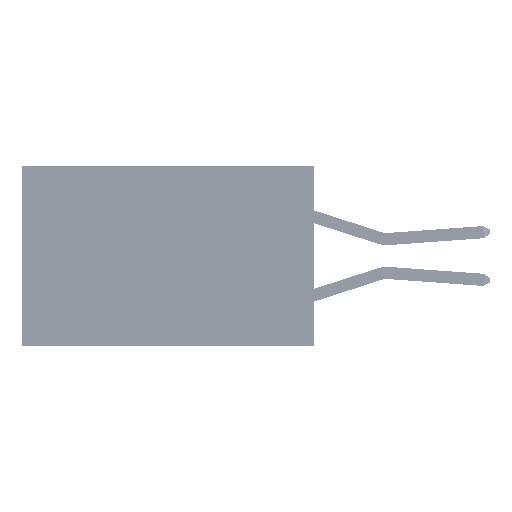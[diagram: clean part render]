
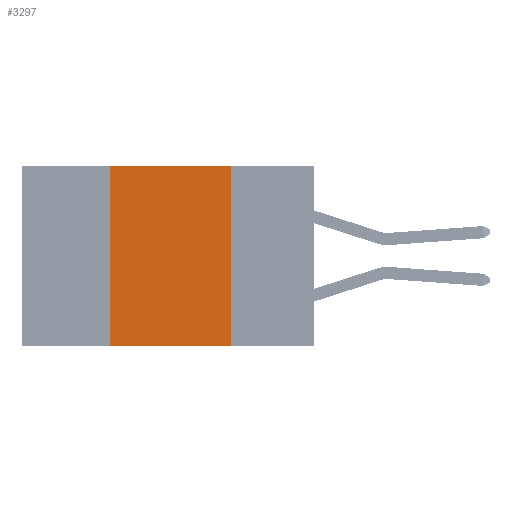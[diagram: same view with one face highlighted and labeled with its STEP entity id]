
A CAD part, left-side view. The second image highlights one B-rep face of the part: STEP entity #3297.
In plain terms, the highlighted planar face has unit normal (-1, 0, 0).
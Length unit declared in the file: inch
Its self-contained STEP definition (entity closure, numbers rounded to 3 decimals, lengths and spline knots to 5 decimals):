
#496 = VERTEX_POINT ( 'NONE', #41765 ) ;
#2485 = LINE ( 'NONE', #27630, #9395 ) ;
#3297 = ADVANCED_FACE ( 'NONE', ( #25194 ), #3970, .F. ) ;
#3970 = PLANE ( 'NONE',  #14318 ) ;
#4510 = EDGE_CURVE ( 'NONE', #26549, #33188, #2485, .T. ) ;
#5505 = DIRECTION ( 'NONE',  ( 0., 0., 1. ) ) ;
#6115 = VECTOR ( 'NONE', #41672, 39.37008 ) ;
#6637 = VERTEX_POINT ( 'NONE', #23015 ) ;
#9395 = VECTOR ( 'NONE', #11869, 39.37008 ) ;
#11869 = DIRECTION ( 'NONE',  ( 0., 0., -1. ) ) ;
#12381 = CARTESIAN_POINT ( 'NONE',  ( 0., 0.17, -0.37 ) ) ;
#12688 = ORIENTED_EDGE ( 'NONE', *, *, #4510, .F. ) ;
#14318 = AXIS2_PLACEMENT_3D ( 'NONE', #44215, #23785, #43866 ) ;
#16305 = CARTESIAN_POINT ( 'NONE',  ( 0., 0.6, 0. ) ) ;
#16565 = ORIENTED_EDGE ( 'NONE', *, *, #43771, .F. ) ;
#23015 = CARTESIAN_POINT ( 'NONE',  ( 0., 0.42, 0. ) ) ;
#23785 = DIRECTION ( 'NONE',  ( 1., 0., 0. ) ) ;
#25194 = FACE_OUTER_BOUND ( 'NONE', #34445, .T. ) ;
#26549 = VERTEX_POINT ( 'NONE', #41019 ) ;
#27255 = EDGE_CURVE ( 'NONE', #496, #33188, #41961, .T. ) ;
#27630 = CARTESIAN_POINT ( 'NONE',  ( 0., 0.17, 0. ) ) ;
#27807 = ORIENTED_EDGE ( 'NONE', *, *, #35668, .F. ) ;
#28914 = DIRECTION ( 'NONE',  ( 0., -1., 0. ) ) ;
#29869 = CARTESIAN_POINT ( 'NONE',  ( 0., 0.42, 0. ) ) ;
#33188 = VERTEX_POINT ( 'NONE', #12381 ) ;
#34445 = EDGE_LOOP ( 'NONE', ( #12688, #27807, #16565, #39528 ) ) ;
#35668 = EDGE_CURVE ( 'NONE', #6637, #26549, #41011, .T. ) ;
#39325 = VECTOR ( 'NONE', #5505, 39.37008 ) ;
#39528 = ORIENTED_EDGE ( 'NONE', *, *, #27255, .T. ) ;
#39980 = LINE ( 'NONE', #29869, #39325 ) ;
#41011 = LINE ( 'NONE', #16305, #44832 ) ;
#41019 = CARTESIAN_POINT ( 'NONE',  ( 0., 0.17, 0. ) ) ;
#41672 = DIRECTION ( 'NONE',  ( 0., -1., 0. ) ) ;
#41765 = CARTESIAN_POINT ( 'NONE',  ( 0., 0.42, -0.37 ) ) ;
#41961 = LINE ( 'NONE', #49450, #6115 ) ;
#43771 = EDGE_CURVE ( 'NONE', #496, #6637, #39980, .T. ) ;
#43866 = DIRECTION ( 'NONE',  ( 0., 0., -1. ) ) ;
#44215 = CARTESIAN_POINT ( 'NONE',  ( 0., 0.6, 0. ) ) ;
#44832 = VECTOR ( 'NONE', #28914, 39.37008 ) ;
#49450 = CARTESIAN_POINT ( 'NONE',  ( 0., 0.6, -0.37 ) ) ;
